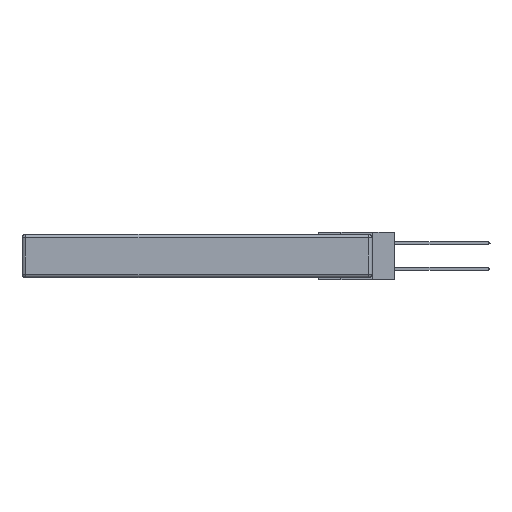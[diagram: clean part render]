
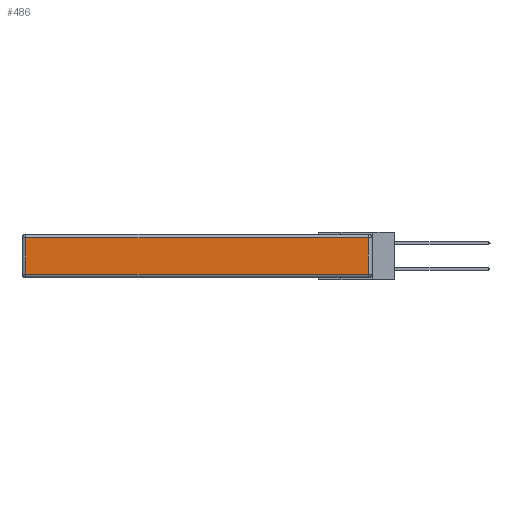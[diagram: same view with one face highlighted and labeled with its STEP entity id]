
A CAD part, left-side view. The second image highlights one B-rep face of the part: STEP entity #486.
In plain terms, the highlighted planar face has unit normal (-1, 0, 0).
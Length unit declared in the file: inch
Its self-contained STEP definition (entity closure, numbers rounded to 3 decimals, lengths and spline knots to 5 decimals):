
#486 = ADVANCED_FACE ( 'NONE', ( #10703 ), #22708, .T. ) ;
#745 = DIRECTION ( 'NONE',  ( -1., 0., 0. ) ) ;
#1909 = ORIENTED_EDGE ( 'NONE', *, *, #34368, .T. ) ;
#2177 = VECTOR ( 'NONE', #16238, 39.37008 ) ;
#2554 = LINE ( 'NONE', #27688, #26540 ) ;
#3265 = CARTESIAN_POINT ( 'NONE',  ( 0., 0., -0.343 ) ) ;
#3434 = VECTOR ( 'NONE', #7455, 39.37008 ) ;
#4431 = VERTEX_POINT ( 'NONE', #17652 ) ;
#5954 = EDGE_CURVE ( 'NONE', #32309, #33593, #7295, .T. ) ;
#7295 = LINE ( 'NONE', #23762, #3434 ) ;
#7455 = DIRECTION ( 'NONE',  ( 0., 0., -1. ) ) ;
#9868 = LINE ( 'NONE', #32602, #2177 ) ;
#10703 = FACE_OUTER_BOUND ( 'NONE', #24204, .T. ) ;
#11181 = DIRECTION ( 'NONE',  ( 0., 0., 1. ) ) ;
#12477 = CARTESIAN_POINT ( 'NONE',  ( 0., 2.72, -0.313 ) ) ;
#12566 = EDGE_CURVE ( 'NONE', #33593, #13628, #32677, .T. ) ;
#13628 = VERTEX_POINT ( 'NONE', #28407 ) ;
#13956 = DIRECTION ( 'NONE',  ( 0., 0., 1. ) ) ;
#14370 = DIRECTION ( 'NONE',  ( 0., -1., 0. ) ) ;
#14484 = CARTESIAN_POINT ( 'NONE',  ( 0., 0., -0.313 ) ) ;
#16238 = DIRECTION ( 'NONE',  ( 0., 1., 0. ) ) ;
#17652 = CARTESIAN_POINT ( 'NONE',  ( 0., 0.03, -0.03 ) ) ;
#22708 = PLANE ( 'NONE',  #27933 ) ;
#23301 = VECTOR ( 'NONE', #14370, 39.37008 ) ;
#23762 = CARTESIAN_POINT ( 'NONE',  ( 0., 2.72, -0.343 ) ) ;
#24204 = EDGE_LOOP ( 'NONE', ( #27867, #34615, #1909, #27833 ) ) ;
#26540 = VECTOR ( 'NONE', #11181, 39.37008 ) ;
#27688 = CARTESIAN_POINT ( 'NONE',  ( 0., 0.03, -0.343 ) ) ;
#27833 = ORIENTED_EDGE ( 'NONE', *, *, #5954, .T. ) ;
#27867 = ORIENTED_EDGE ( 'NONE', *, *, #12566, .T. ) ;
#27933 = AXIS2_PLACEMENT_3D ( 'NONE', #3265, #745, #13956 ) ;
#28407 = CARTESIAN_POINT ( 'NONE',  ( 0., 0.03, -0.313 ) ) ;
#29556 = EDGE_CURVE ( 'NONE', #13628, #4431, #2554, .T. ) ;
#31531 = CARTESIAN_POINT ( 'NONE',  ( 0., 2.72, -0.03 ) ) ;
#32309 = VERTEX_POINT ( 'NONE', #31531 ) ;
#32602 = CARTESIAN_POINT ( 'NONE',  ( 0., 2.75, -0.03 ) ) ;
#32677 = LINE ( 'NONE', #14484, #23301 ) ;
#33593 = VERTEX_POINT ( 'NONE', #12477 ) ;
#34368 = EDGE_CURVE ( 'NONE', #4431, #32309, #9868, .T. ) ;
#34615 = ORIENTED_EDGE ( 'NONE', *, *, #29556, .T. ) ;
